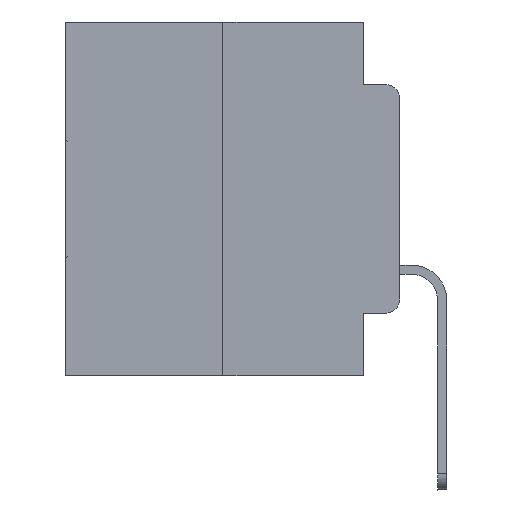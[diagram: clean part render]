
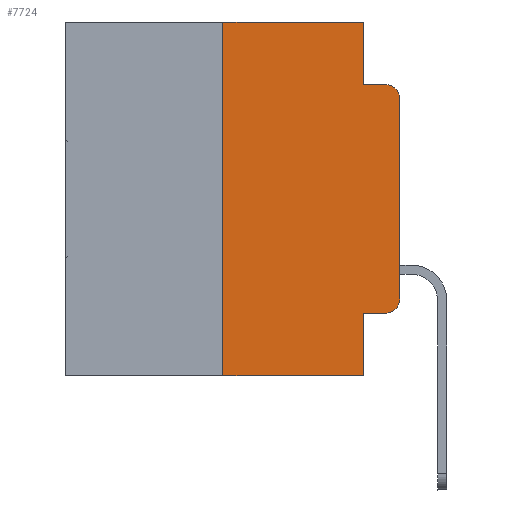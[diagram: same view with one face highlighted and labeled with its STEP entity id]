
A CAD part, left-side view. The second image highlights one B-rep face of the part: STEP entity #7724.
In plain terms, the highlighted planar face has unit normal (-1, 0, 0).
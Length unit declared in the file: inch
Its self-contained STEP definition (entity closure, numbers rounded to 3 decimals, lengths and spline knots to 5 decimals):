
#316 = CARTESIAN_POINT ( 'NONE',  ( 0., 0., -0.3915 ) ) ;
#375 = VERTEX_POINT ( 'NONE', #316 ) ;
#396 = VECTOR ( 'NONE', #17579, 39.37008 ) ;
#2321 = DIRECTION ( 'NONE',  ( 0., 0., -1. ) ) ;
#2343 = CARTESIAN_POINT ( 'NONE',  ( 0., 0.25, 0. ) ) ;
#2745 = CIRCLE ( 'NONE', #7719, 0.02 ) ;
#2856 = DIRECTION ( 'NONE',  ( -1., 0., 0. ) ) ;
#2939 = CARTESIAN_POINT ( 'NONE',  ( 0., 0.02, -0.4115 ) ) ;
#3025 = VERTEX_POINT ( 'NONE', #19217 ) ;
#3455 = CARTESIAN_POINT ( 'NONE',  ( 0., 0., 0. ) ) ;
#3961 = ORIENTED_EDGE ( 'NONE', *, *, #5863, .T. ) ;
#4983 = DIRECTION ( 'NONE',  ( 0., 0., -1. ) ) ;
#5863 = EDGE_CURVE ( 'NONE', #375, #17671, #18243, .T. ) ;
#6126 = FACE_OUTER_BOUND ( 'NONE', #10730, .T. ) ;
#6153 = CARTESIAN_POINT ( 'NONE',  ( 0., 0.051, -0.0885 ) ) ;
#6431 = CARTESIAN_POINT ( 'NONE',  ( 0., 0.051, 0. ) ) ;
#6496 = CARTESIAN_POINT ( 'NONE',  ( 0., 0.25, 0. ) ) ;
#6570 = DIRECTION ( 'NONE',  ( 0., 0., -1. ) ) ;
#7392 = EDGE_CURVE ( 'NONE', #9602, #3025, #8855, .T. ) ;
#7571 = VERTEX_POINT ( 'NONE', #24880 ) ;
#7719 = AXIS2_PLACEMENT_3D ( 'NONE', #15921, #20176, #4983 ) ;
#7724 = ADVANCED_FACE ( 'NONE', ( #6126 ), #14494, .F. ) ;
#7731 = ORIENTED_EDGE ( 'NONE', *, *, #10898, .F. ) ;
#7891 = LINE ( 'NONE', #14556, #18501 ) ;
#8174 = DIRECTION ( 'NONE',  ( 0., -1., 0. ) ) ;
#8467 = ORIENTED_EDGE ( 'NONE', *, *, #24997, .F. ) ;
#8538 = DIRECTION ( 'NONE',  ( 0., -1., 0. ) ) ;
#8653 = VECTOR ( 'NONE', #2321, 39.37008 ) ;
#8718 = VERTEX_POINT ( 'NONE', #10121 ) ;
#8855 = LINE ( 'NONE', #6431, #24042 ) ;
#9602 = VERTEX_POINT ( 'NONE', #18984 ) ;
#9878 = ORIENTED_EDGE ( 'NONE', *, *, #10329, .T. ) ;
#10121 = CARTESIAN_POINT ( 'NONE',  ( 0., 0.051, -0.5 ) ) ;
#10329 = EDGE_CURVE ( 'NONE', #17671, #24416, #2745, .T. ) ;
#10545 = ORIENTED_EDGE ( 'NONE', *, *, #7392, .F. ) ;
#10730 = EDGE_LOOP ( 'NONE', ( #3961, #9878, #11574, #10545, #7731, #11866, #25787, #8467, #24224, #11107 ) ) ;
#10898 = EDGE_CURVE ( 'NONE', #27238, #9602, #10953, .T. ) ;
#10953 = LINE ( 'NONE', #19471, #27175 ) ;
#11107 = ORIENTED_EDGE ( 'NONE', *, *, #11159, .T. ) ;
#11159 = EDGE_CURVE ( 'NONE', #14991, #375, #23571, .T. ) ;
#11574 = ORIENTED_EDGE ( 'NONE', *, *, #24871, .F. ) ;
#11866 = ORIENTED_EDGE ( 'NONE', *, *, #23080, .F. ) ;
#12231 = VECTOR ( 'NONE', #17577, 39.37008 ) ;
#12819 = DIRECTION ( 'NONE',  ( 0., -1., 0. ) ) ;
#13435 = LINE ( 'NONE', #15432, #12231 ) ;
#13634 = CARTESIAN_POINT ( 'NONE',  ( 0., 0.02, -0.3915 ) ) ;
#13958 = DIRECTION ( 'NONE',  ( 0., 0., 1. ) ) ;
#14494 = PLANE ( 'NONE',  #24133 ) ;
#14556 = CARTESIAN_POINT ( 'NONE',  ( 0., 0.051, -0.4115 ) ) ;
#14991 = VERTEX_POINT ( 'NONE', #2939 ) ;
#15432 = CARTESIAN_POINT ( 'NONE',  ( 0., 0.473, -0.5 ) ) ;
#15583 = LINE ( 'NONE', #6496, #396 ) ;
#15919 = DIRECTION ( 'NONE',  ( 0., 0., -1. ) ) ;
#15921 = CARTESIAN_POINT ( 'NONE',  ( 0., 0.02, -0.1085 ) ) ;
#17274 = CARTESIAN_POINT ( 'NONE',  ( 0., 0.02, -0.0885 ) ) ;
#17575 = CARTESIAN_POINT ( 'NONE',  ( 0., 0.25, -0.5 ) ) ;
#17577 = DIRECTION ( 'NONE',  ( 0., -1., 0. ) ) ;
#17579 = DIRECTION ( 'NONE',  ( 0., 0., 1. ) ) ;
#17671 = VERTEX_POINT ( 'NONE', #21238 ) ;
#18243 = LINE ( 'NONE', #3455, #21476 ) ;
#18501 = VECTOR ( 'NONE', #8174, 39.37008 ) ;
#18984 = CARTESIAN_POINT ( 'NONE',  ( 0., 0.051, 0. ) ) ;
#19217 = CARTESIAN_POINT ( 'NONE',  ( 0., 0.051, -0.0885 ) ) ;
#19471 = CARTESIAN_POINT ( 'NONE',  ( 0., 0.473, 0. ) ) ;
#19478 = AXIS2_PLACEMENT_3D ( 'NONE', #13634, #2856, #15919 ) ;
#20176 = DIRECTION ( 'NONE',  ( -1., 0., 0. ) ) ;
#21238 = CARTESIAN_POINT ( 'NONE',  ( 0., 0., -0.1085 ) ) ;
#21476 = VECTOR ( 'NONE', #13958, 39.37008 ) ;
#22041 = LINE ( 'NONE', #26159, #8653 ) ;
#22895 = DIRECTION ( 'NONE',  ( 0., 0., -1. ) ) ;
#22955 = EDGE_CURVE ( 'NONE', #26885, #8718, #13435, .T. ) ;
#23080 = EDGE_CURVE ( 'NONE', #26885, #27238, #15583, .T. ) ;
#23571 = CIRCLE ( 'NONE', #19478, 0.02 ) ;
#24042 = VECTOR ( 'NONE', #6570, 39.37008 ) ;
#24133 = AXIS2_PLACEMENT_3D ( 'NONE', #25161, #27695, #22895 ) ;
#24224 = ORIENTED_EDGE ( 'NONE', *, *, #27034, .T. ) ;
#24416 = VERTEX_POINT ( 'NONE', #17274 ) ;
#24871 = EDGE_CURVE ( 'NONE', #3025, #24416, #25607, .T. ) ;
#24880 = CARTESIAN_POINT ( 'NONE',  ( 0., 0.051, -0.4115 ) ) ;
#24997 = EDGE_CURVE ( 'NONE', #7571, #8718, #22041, .T. ) ;
#25161 = CARTESIAN_POINT ( 'NONE',  ( 0., 0.473, 0. ) ) ;
#25607 = LINE ( 'NONE', #6153, #25850 ) ;
#25787 = ORIENTED_EDGE ( 'NONE', *, *, #22955, .T. ) ;
#25850 = VECTOR ( 'NONE', #12819, 39.37008 ) ;
#26159 = CARTESIAN_POINT ( 'NONE',  ( 0., 0.051, 0. ) ) ;
#26885 = VERTEX_POINT ( 'NONE', #17575 ) ;
#27034 = EDGE_CURVE ( 'NONE', #7571, #14991, #7891, .T. ) ;
#27175 = VECTOR ( 'NONE', #8538, 39.37008 ) ;
#27238 = VERTEX_POINT ( 'NONE', #2343 ) ;
#27695 = DIRECTION ( 'NONE',  ( 1., 0., 0. ) ) ;
